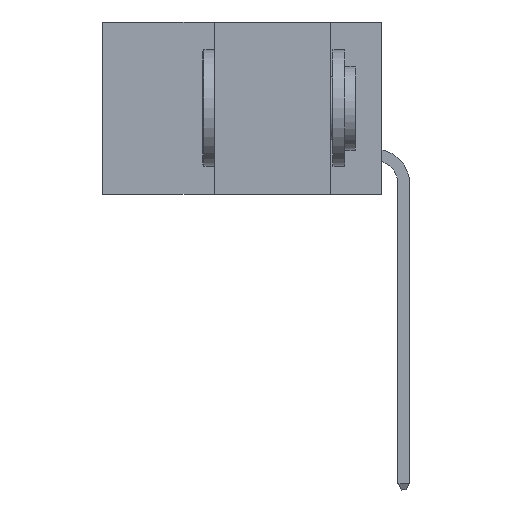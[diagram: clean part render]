
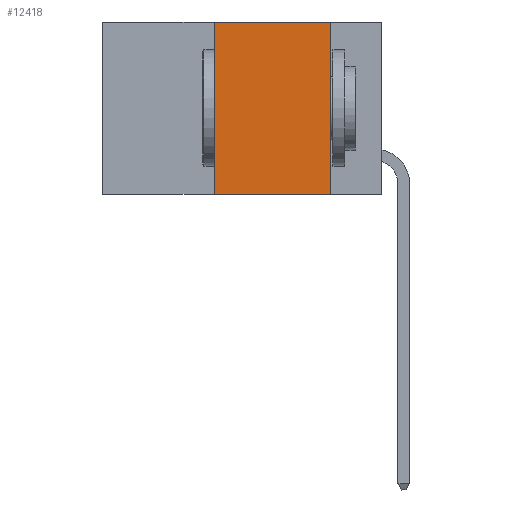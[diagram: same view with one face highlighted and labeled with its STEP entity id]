
A CAD part, left-side view. The second image highlights one B-rep face of the part: STEP entity #12418.
In plain terms, the highlighted planar face has unit normal (-1, 0, 0).
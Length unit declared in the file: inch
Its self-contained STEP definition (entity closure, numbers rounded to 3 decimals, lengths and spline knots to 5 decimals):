
#39 = DIRECTION ( 'NONE',  ( 0., -1., 0. ) ) ;
#1124 = DIRECTION ( 'NONE',  ( 0., 0., -1. ) ) ;
#2308 = CARTESIAN_POINT ( 'NONE',  ( 0., 0.36, 0. ) ) ;
#3362 = EDGE_CURVE ( 'NONE', #13464, #22025, #37219, .T. ) ;
#4253 = EDGE_LOOP ( 'NONE', ( #12510, #26410, #8328, #11731 ) ) ;
#4993 = VECTOR ( 'NONE', #39, 39.37008 ) ;
#5694 = CARTESIAN_POINT ( 'NONE',  ( 0., 0.36, -0.37 ) ) ;
#6784 = PLANE ( 'NONE',  #23895 ) ;
#8328 = ORIENTED_EDGE ( 'NONE', *, *, #3362, .F. ) ;
#8938 = EDGE_CURVE ( 'NONE', #22025, #32125, #11405, .T. ) ;
#11405 = LINE ( 'NONE', #23472, #33564 ) ;
#11731 = ORIENTED_EDGE ( 'NONE', *, *, #20277, .T. ) ;
#11824 = DIRECTION ( 'NONE',  ( 0., -1., 0. ) ) ;
#12418 = ADVANCED_FACE ( 'NONE', ( #26371 ), #6784, .F. ) ;
#12510 = ORIENTED_EDGE ( 'NONE', *, *, #20488, .F. ) ;
#13097 = VECTOR ( 'NONE', #18461, 39.37008 ) ;
#13464 = VERTEX_POINT ( 'NONE', #5694 ) ;
#13582 = LINE ( 'NONE', #14416, #4993 ) ;
#14416 = CARTESIAN_POINT ( 'NONE',  ( 0., 0.6, -0.37 ) ) ;
#16547 = DIRECTION ( 'NONE',  ( 0., 0., 1. ) ) ;
#17208 = VERTEX_POINT ( 'NONE', #35591 ) ;
#17776 = CARTESIAN_POINT ( 'NONE',  ( 0., 0.11, 0. ) ) ;
#18432 = DIRECTION ( 'NONE',  ( 1., 0., 0. ) ) ;
#18461 = DIRECTION ( 'NONE',  ( 0., 0., -1. ) ) ;
#20277 = EDGE_CURVE ( 'NONE', #13464, #17208, #13582, .T. ) ;
#20488 = EDGE_CURVE ( 'NONE', #32125, #17208, #36193, .T. ) ;
#22025 = VERTEX_POINT ( 'NONE', #2308 ) ;
#23472 = CARTESIAN_POINT ( 'NONE',  ( 0., 0.6, 0. ) ) ;
#23895 = AXIS2_PLACEMENT_3D ( 'NONE', #35722, #18432, #1124 ) ;
#26371 = FACE_OUTER_BOUND ( 'NONE', #4253, .T. ) ;
#26410 = ORIENTED_EDGE ( 'NONE', *, *, #8938, .F. ) ;
#28086 = CARTESIAN_POINT ( 'NONE',  ( 0., 0.36, 0. ) ) ;
#29572 = VECTOR ( 'NONE', #16547, 39.37008 ) ;
#29986 = CARTESIAN_POINT ( 'NONE',  ( 0., 0.11, 0. ) ) ;
#32125 = VERTEX_POINT ( 'NONE', #17776 ) ;
#33564 = VECTOR ( 'NONE', #11824, 39.37008 ) ;
#35591 = CARTESIAN_POINT ( 'NONE',  ( 0., 0.11, -0.37 ) ) ;
#35722 = CARTESIAN_POINT ( 'NONE',  ( 0., 0.6, 0. ) ) ;
#36193 = LINE ( 'NONE', #29986, #13097 ) ;
#37219 = LINE ( 'NONE', #28086, #29572 ) ;
